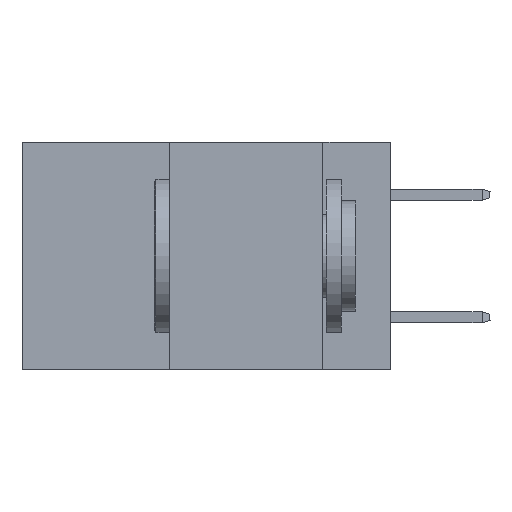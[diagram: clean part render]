
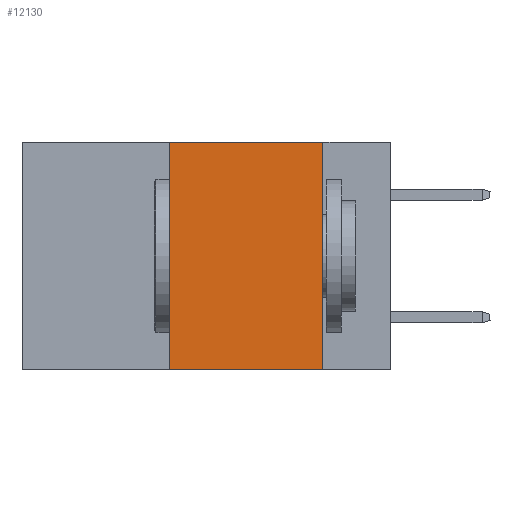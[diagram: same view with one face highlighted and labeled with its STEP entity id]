
A CAD part, left-side view. The second image highlights one B-rep face of the part: STEP entity #12130.
In plain terms, the highlighted planar face has unit normal (-1, 0, 0).
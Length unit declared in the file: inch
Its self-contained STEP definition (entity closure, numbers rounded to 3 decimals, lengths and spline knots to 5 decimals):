
#138 = DIRECTION ( 'NONE',  ( 0., 0., -1. ) ) ;
#1588 = AXIS2_PLACEMENT_3D ( 'NONE', #32278, #8053, #138 ) ;
#2247 = EDGE_CURVE ( 'NONE', #18109, #15336, #33398, .T. ) ;
#3417 = CARTESIAN_POINT ( 'NONE',  ( 0., 0.11, -0.37 ) ) ;
#4457 = FACE_OUTER_BOUND ( 'NONE', #30986, .T. ) ;
#8053 = DIRECTION ( 'NONE',  ( 1., 0., 0. ) ) ;
#9009 = DIRECTION ( 'NONE',  ( 0., -1., 0. ) ) ;
#10490 = PLANE ( 'NONE',  #1588 ) ;
#11183 = VECTOR ( 'NONE', #26951, 39.37008 ) ;
#12130 = ADVANCED_FACE ( 'NONE', ( #4457 ), #10490, .F. ) ;
#14433 = ORIENTED_EDGE ( 'NONE', *, *, #18555, .T. ) ;
#15125 = EDGE_CURVE ( 'NONE', #20302, #18109, #29508, .T. ) ;
#15216 = EDGE_CURVE ( 'NONE', #20742, #20302, #25365, .T. ) ;
#15336 = VERTEX_POINT ( 'NONE', #3417 ) ;
#15495 = DIRECTION ( 'NONE',  ( 0., -1., 0. ) ) ;
#16166 = VECTOR ( 'NONE', #15495, 39.37008 ) ;
#16390 = LINE ( 'NONE', #32901, #33101 ) ;
#18109 = VERTEX_POINT ( 'NONE', #33729 ) ;
#18555 = EDGE_CURVE ( 'NONE', #20742, #15336, #16390, .T. ) ;
#20302 = VERTEX_POINT ( 'NONE', #21022 ) ;
#20637 = ORIENTED_EDGE ( 'NONE', *, *, #15216, .F. ) ;
#20742 = VERTEX_POINT ( 'NONE', #26247 ) ;
#21022 = CARTESIAN_POINT ( 'NONE',  ( 0., 0.36, 0. ) ) ;
#22562 = DIRECTION ( 'NONE',  ( 0., 0., -1. ) ) ;
#25365 = LINE ( 'NONE', #29490, #11183 ) ;
#26247 = CARTESIAN_POINT ( 'NONE',  ( 0., 0.36, -0.37 ) ) ;
#26336 = VECTOR ( 'NONE', #22562, 39.37008 ) ;
#26951 = DIRECTION ( 'NONE',  ( 0., 0., 1. ) ) ;
#28759 = ORIENTED_EDGE ( 'NONE', *, *, #15125, .F. ) ;
#29490 = CARTESIAN_POINT ( 'NONE',  ( 0., 0.36, 0. ) ) ;
#29508 = LINE ( 'NONE', #31489, #16166 ) ;
#30483 = CARTESIAN_POINT ( 'NONE',  ( 0., 0.11, 0. ) ) ;
#30969 = ORIENTED_EDGE ( 'NONE', *, *, #2247, .F. ) ;
#30986 = EDGE_LOOP ( 'NONE', ( #30969, #28759, #20637, #14433 ) ) ;
#31489 = CARTESIAN_POINT ( 'NONE',  ( 0., 0.6, 0. ) ) ;
#32278 = CARTESIAN_POINT ( 'NONE',  ( 0., 0.6, 0. ) ) ;
#32901 = CARTESIAN_POINT ( 'NONE',  ( 0., 0.6, -0.37 ) ) ;
#33101 = VECTOR ( 'NONE', #9009, 39.37008 ) ;
#33398 = LINE ( 'NONE', #30483, #26336 ) ;
#33729 = CARTESIAN_POINT ( 'NONE',  ( 0., 0.11, 0. ) ) ;
